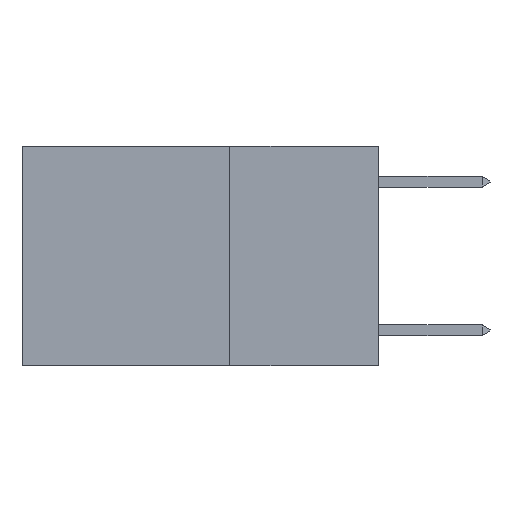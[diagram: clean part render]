
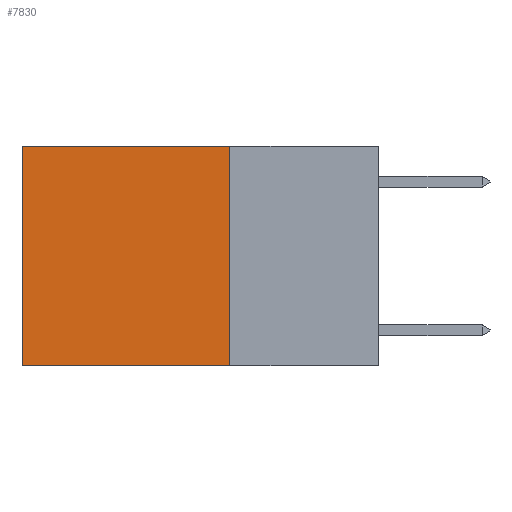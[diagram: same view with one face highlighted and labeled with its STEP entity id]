
A CAD part, left-side view. The second image highlights one B-rep face of the part: STEP entity #7830.
In plain terms, the highlighted planar face has unit normal (-1, 0, 0).
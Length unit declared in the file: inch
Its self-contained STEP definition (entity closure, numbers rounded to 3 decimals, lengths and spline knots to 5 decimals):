
#685 = CARTESIAN_POINT ( 'NONE',  ( 0.2625, 0.25, 0. ) ) ;
#902 = VECTOR ( 'NONE', #2583, 39.37008 ) ;
#934 = LINE ( 'NONE', #16609, #12910 ) ;
#1965 = ORIENTED_EDGE ( 'NONE', *, *, #3157, .T. ) ;
#2583 = DIRECTION ( 'NONE',  ( 0., 1., 0. ) ) ;
#2746 = CARTESIAN_POINT ( 'NONE',  ( 0.2625, 0.25, 0. ) ) ;
#3061 = DIRECTION ( 'NONE',  ( 1., 0., 0. ) ) ;
#3157 = EDGE_CURVE ( 'NONE', #13007, #3280, #15007, .T. ) ;
#3280 = VERTEX_POINT ( 'NONE', #15175 ) ;
#4157 = PLANE ( 'NONE',  #14262 ) ;
#4968 = EDGE_CURVE ( 'NONE', #11065, #3280, #934, .T. ) ;
#5026 = DIRECTION ( 'NONE',  ( 0., 0., -1. ) ) ;
#5030 = VERTEX_POINT ( 'NONE', #8836 ) ;
#5783 = EDGE_LOOP ( 'NONE', ( #1965, #10489, #15724, #14502 ) ) ;
#6880 = VECTOR ( 'NONE', #12444, 39.37008 ) ;
#7327 = EDGE_CURVE ( 'NONE', #5030, #13007, #14259, .T. ) ;
#7830 = ADVANCED_FACE ( 'NONE', ( #14912 ), #4157, .F. ) ;
#8088 = CARTESIAN_POINT ( 'NONE',  ( 0.2625, 0.6, 0. ) ) ;
#8339 = CARTESIAN_POINT ( 'NONE',  ( 0.2625, 0.6, 0. ) ) ;
#8609 = VECTOR ( 'NONE', #5026, 39.37008 ) ;
#8753 = DIRECTION ( 'NONE',  ( 0., 1., 0. ) ) ;
#8836 = CARTESIAN_POINT ( 'NONE',  ( 0.2625, 0.25, 0. ) ) ;
#10489 = ORIENTED_EDGE ( 'NONE', *, *, #4968, .F. ) ;
#11017 = CARTESIAN_POINT ( 'NONE',  ( 0.2625, 0.25, -0.37 ) ) ;
#11065 = VERTEX_POINT ( 'NONE', #11017 ) ;
#12444 = DIRECTION ( 'NONE',  ( 0., 0., -1. ) ) ;
#12910 = VECTOR ( 'NONE', #8753, 39.37008 ) ;
#13007 = VERTEX_POINT ( 'NONE', #8088 ) ;
#13642 = DIRECTION ( 'NONE',  ( 0., 0., -1. ) ) ;
#14259 = LINE ( 'NONE', #2746, #902 ) ;
#14262 = AXIS2_PLACEMENT_3D ( 'NONE', #685, #3061, #13642 ) ;
#14502 = ORIENTED_EDGE ( 'NONE', *, *, #7327, .T. ) ;
#14912 = FACE_OUTER_BOUND ( 'NONE', #5783, .T. ) ;
#15007 = LINE ( 'NONE', #8339, #6880 ) ;
#15175 = CARTESIAN_POINT ( 'NONE',  ( 0.2625, 0.6, -0.37 ) ) ;
#15441 = LINE ( 'NONE', #16800, #8609 ) ;
#15574 = EDGE_CURVE ( 'NONE', #5030, #11065, #15441, .T. ) ;
#15724 = ORIENTED_EDGE ( 'NONE', *, *, #15574, .F. ) ;
#16609 = CARTESIAN_POINT ( 'NONE',  ( 0.2625, 0.25, -0.37 ) ) ;
#16800 = CARTESIAN_POINT ( 'NONE',  ( 0.2625, 0.25, 0. ) ) ;
